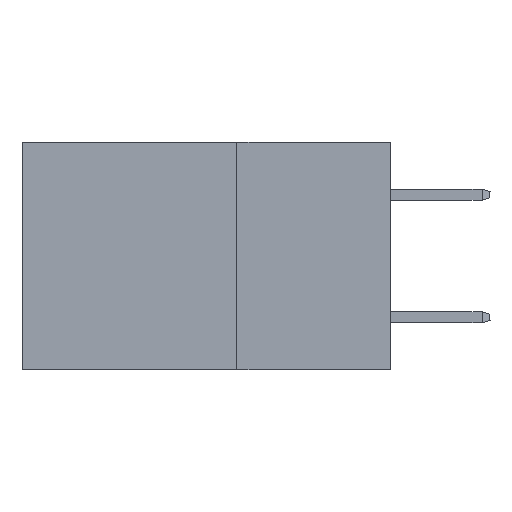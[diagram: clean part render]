
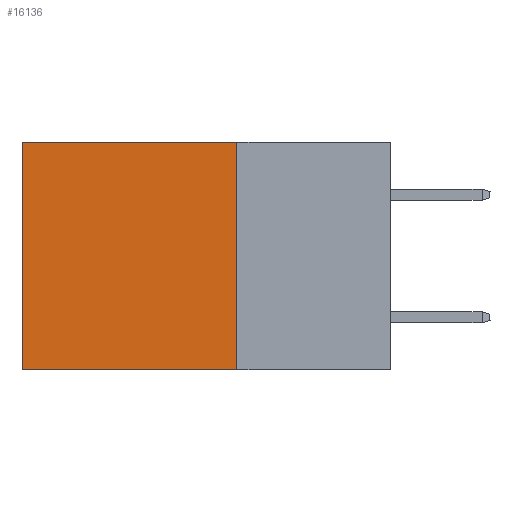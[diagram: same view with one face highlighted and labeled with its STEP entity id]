
A CAD part, left-side view. The second image highlights one B-rep face of the part: STEP entity #16136.
In plain terms, the highlighted planar face has unit normal (-1, 0, 0).
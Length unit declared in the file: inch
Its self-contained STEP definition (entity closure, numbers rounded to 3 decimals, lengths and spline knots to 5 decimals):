
#553 = DIRECTION ( 'NONE',  ( 0., 0., -1. ) ) ;
#657 = PLANE ( 'NONE',  #709 ) ;
#709 = AXIS2_PLACEMENT_3D ( 'NONE', #11099, #9871, #2031 ) ;
#1629 = ORIENTED_EDGE ( 'NONE', *, *, #12497, .T. ) ;
#2031 = DIRECTION ( 'NONE',  ( 0., 0., -1. ) ) ;
#2619 = VECTOR ( 'NONE', #8736, 39.37008 ) ;
#5299 = CARTESIAN_POINT ( 'NONE',  ( 0.2875, 0.6, -0.37 ) ) ;
#5301 = CARTESIAN_POINT ( 'NONE',  ( 0.2875, 0.25, -0.37 ) ) ;
#5897 = LINE ( 'NONE', #16004, #15517 ) ;
#7381 = VERTEX_POINT ( 'NONE', #5299 ) ;
#8085 = LINE ( 'NONE', #8505, #8490 ) ;
#8097 = ORIENTED_EDGE ( 'NONE', *, *, #9957, .F. ) ;
#8316 = CARTESIAN_POINT ( 'NONE',  ( 0.2875, 0.25, -0.37 ) ) ;
#8490 = VECTOR ( 'NONE', #553, 39.37008 ) ;
#8505 = CARTESIAN_POINT ( 'NONE',  ( 0.2875, 0.25, 0. ) ) ;
#8535 = DIRECTION ( 'NONE',  ( 0., 0., -1. ) ) ;
#8671 = EDGE_CURVE ( 'NONE', #12127, #7381, #10492, .T. ) ;
#8736 = DIRECTION ( 'NONE',  ( 0., 1., 0. ) ) ;
#8749 = EDGE_CURVE ( 'NONE', #9646, #7381, #5897, .T. ) ;
#8804 = EDGE_LOOP ( 'NONE', ( #11376, #11000, #8097, #1629 ) ) ;
#9432 = FACE_OUTER_BOUND ( 'NONE', #8804, .T. ) ;
#9585 = LINE ( 'NONE', #14954, #2619 ) ;
#9646 = VERTEX_POINT ( 'NONE', #14186 ) ;
#9871 = DIRECTION ( 'NONE',  ( 1., 0., 0. ) ) ;
#9957 = EDGE_CURVE ( 'NONE', #12132, #12127, #8085, .T. ) ;
#10414 = CARTESIAN_POINT ( 'NONE',  ( 0.2875, 0.25, 0. ) ) ;
#10492 = LINE ( 'NONE', #8316, #16678 ) ;
#11000 = ORIENTED_EDGE ( 'NONE', *, *, #8671, .F. ) ;
#11099 = CARTESIAN_POINT ( 'NONE',  ( 0.2875, 0.25, 0. ) ) ;
#11376 = ORIENTED_EDGE ( 'NONE', *, *, #8749, .T. ) ;
#12127 = VERTEX_POINT ( 'NONE', #5301 ) ;
#12132 = VERTEX_POINT ( 'NONE', #10414 ) ;
#12497 = EDGE_CURVE ( 'NONE', #12132, #9646, #9585, .T. ) ;
#14186 = CARTESIAN_POINT ( 'NONE',  ( 0.2875, 0.6, 0. ) ) ;
#14593 = DIRECTION ( 'NONE',  ( 0., 1., 0. ) ) ;
#14954 = CARTESIAN_POINT ( 'NONE',  ( 0.2875, 0.25, 0. ) ) ;
#15517 = VECTOR ( 'NONE', #8535, 39.37008 ) ;
#16004 = CARTESIAN_POINT ( 'NONE',  ( 0.2875, 0.6, 0. ) ) ;
#16136 = ADVANCED_FACE ( 'NONE', ( #9432 ), #657, .F. ) ;
#16678 = VECTOR ( 'NONE', #14593, 39.37008 ) ;
